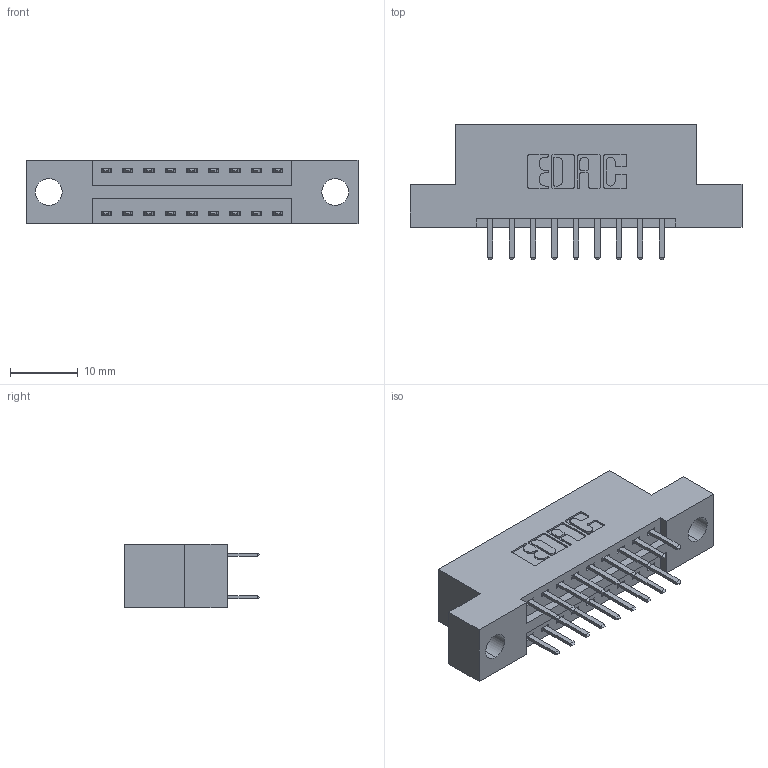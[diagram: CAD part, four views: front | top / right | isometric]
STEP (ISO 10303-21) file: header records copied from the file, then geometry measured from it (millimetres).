
FILE_DESCRIPTION (( 'STEP AP203' ), '1' );
FILE_NAME ('346-018-520-204.STEP', '2022-05-18T16:54:40', ( '' ), ( '' ), 'SwSTEP 2.0', 'SolidWorks 2020', '' );
FILE_SCHEMA (( 'CONFIG_CONTROL_DESIGN' ));
Length unit declared in the file: inch
Products named in the file (3): 346-018-520-204; 345-292-001_345-293-120; 346 Part_Flush Mounting Lugs - 0.156 Dia-TH
Assembly tree (19 placements, depth 2):
  346-018-520-204
    346 Part_Flush Mounting Lugs - 0.156 Dia-TH
    345-292-001_345-293-120  x18
Bounding box: 49.15 x 20.02 x 9.4 mm (x, y, z)
Volume: 4422.5 mm3; surface area: 5389.7 mm2
Topology: 19 solids, 19 shells, 1144 faces, 3299 edges, 2150 vertices
Faces by surface type: plane 756, cylinder 388
Entity records: 10849 total; most frequent: CARTESIAN_POINT 1850, ORIENTED_EDGE 1770, DIRECTION 1669, EDGE_CURVE 885, LINE 713, VECTOR 713, VERTEX_POINT 586, AXIS2_PLACEMENT_3D 478
